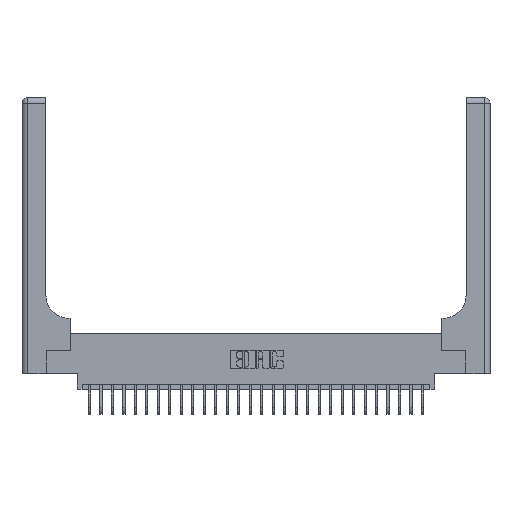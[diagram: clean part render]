
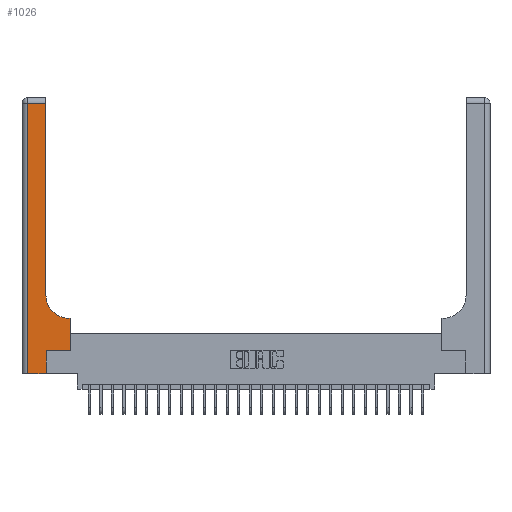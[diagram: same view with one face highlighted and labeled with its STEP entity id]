
A CAD part, top view. The second image highlights one B-rep face of the part: STEP entity #1026.
In plain terms, the highlighted planar face has unit normal (0, 0, 1).
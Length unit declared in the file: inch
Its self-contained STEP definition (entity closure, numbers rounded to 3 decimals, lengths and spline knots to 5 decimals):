
#331 = EDGE_CURVE ( 'NONE', #27107, #9258, #3644, .T. ) ;
#975 = CARTESIAN_POINT ( 'NONE',  ( 0.26, 0.85, 0.37 ) ) ;
#1026 = ADVANCED_FACE ( 'NONE', ( #7082 ), #26937, .F. ) ;
#1306 = CARTESIAN_POINT ( 'NONE',  ( 0.528, 0.25, 0.37 ) ) ;
#1690 = CARTESIAN_POINT ( 'NONE',  ( 0., 2.94, 0.37 ) ) ;
#1977 = DIRECTION ( 'NONE',  ( 0., 1., 0. ) ) ;
#2472 = CARTESIAN_POINT ( 'NONE',  ( 0.265, 0.25, 0.37 ) ) ;
#2735 = ORIENTED_EDGE ( 'NONE', *, *, #331, .T. ) ;
#2894 = ORIENTED_EDGE ( 'NONE', *, *, #18799, .T. ) ;
#2970 = DIRECTION ( 'NONE',  ( -1., 0., 0. ) ) ;
#3071 = EDGE_CURVE ( 'NONE', #18480, #27107, #7790, .T. ) ;
#3644 = CIRCLE ( 'NONE', #4906, 0.25 ) ;
#4906 = AXIS2_PLACEMENT_3D ( 'NONE', #14392, #12033, #23158 ) ;
#5175 = CARTESIAN_POINT ( 'NONE',  ( 0.265, 0., 0.37 ) ) ;
#5927 = VECTOR ( 'NONE', #7418, 39.37008 ) ;
#6182 = VERTEX_POINT ( 'NONE', #6375 ) ;
#6375 = CARTESIAN_POINT ( 'NONE',  ( 0.265, 0., 0.37 ) ) ;
#6427 = CARTESIAN_POINT ( 'NONE',  ( 0.06, 0., 0.37 ) ) ;
#7082 = FACE_OUTER_BOUND ( 'NONE', #8009, .T. ) ;
#7418 = DIRECTION ( 'NONE',  ( 0., 1., 0. ) ) ;
#7531 = DIRECTION ( 'NONE',  ( 0., 0., -1. ) ) ;
#7692 = ORIENTED_EDGE ( 'NONE', *, *, #22414, .T. ) ;
#7784 = LINE ( 'NONE', #23981, #21418 ) ;
#7790 = LINE ( 'NONE', #20280, #20394 ) ;
#7985 = LINE ( 'NONE', #5175, #5927 ) ;
#8009 = EDGE_LOOP ( 'NONE', ( #28107, #18977, #25809, #2894, #25044, #7692, #16005, #24424, #2735 ) ) ;
#8267 = VERTEX_POINT ( 'NONE', #21131 ) ;
#8695 = DIRECTION ( 'NONE',  ( 0., -1., 0. ) ) ;
#9064 = VERTEX_POINT ( 'NONE', #6427 ) ;
#9258 = VERTEX_POINT ( 'NONE', #975 ) ;
#9367 = LINE ( 'NONE', #1690, #11394 ) ;
#9979 = CARTESIAN_POINT ( 'NONE',  ( 0.06, 2.94, 0.37 ) ) ;
#10474 = VECTOR ( 'NONE', #1977, 39.37008 ) ;
#10831 = VERTEX_POINT ( 'NONE', #20837 ) ;
#10921 = DIRECTION ( 'NONE',  ( 1., 0., 0. ) ) ;
#11394 = VECTOR ( 'NONE', #14892, 39.37008 ) ;
#11463 = VERTEX_POINT ( 'NONE', #9979 ) ;
#12001 = EDGE_CURVE ( 'NONE', #9258, #8267, #27906, .T. ) ;
#12033 = DIRECTION ( 'NONE',  ( 0., 0., -1. ) ) ;
#12632 = LINE ( 'NONE', #21747, #21855 ) ;
#13184 = CARTESIAN_POINT ( 'NONE',  ( 0.26, 3., 0.37 ) ) ;
#14049 = EDGE_CURVE ( 'NONE', #6182, #10831, #7985, .T. ) ;
#14392 = CARTESIAN_POINT ( 'NONE',  ( 0.51, 0.85, 0.37 ) ) ;
#14892 = DIRECTION ( 'NONE',  ( -1., 0., 0. ) ) ;
#16005 = ORIENTED_EDGE ( 'NONE', *, *, #27167, .T. ) ;
#16258 = CARTESIAN_POINT ( 'NONE',  ( 0.51, 0.6, 0.37 ) ) ;
#16285 = AXIS2_PLACEMENT_3D ( 'NONE', #18296, #7531, #27121 ) ;
#16824 = DIRECTION ( 'NONE',  ( 0., 1., 0. ) ) ;
#17018 = CARTESIAN_POINT ( 'NONE',  ( 0.528, 0.25, 0.37 ) ) ;
#18296 = CARTESIAN_POINT ( 'NONE',  ( 0., 3., 0.37 ) ) ;
#18480 = VERTEX_POINT ( 'NONE', #23336 ) ;
#18799 = EDGE_CURVE ( 'NONE', #9064, #6182, #7784, .T. ) ;
#18977 = ORIENTED_EDGE ( 'NONE', *, *, #21145, .T. ) ;
#20280 = CARTESIAN_POINT ( 'NONE',  ( 0.26, 0.6, 0.37 ) ) ;
#20394 = VECTOR ( 'NONE', #2970, 39.37008 ) ;
#20837 = CARTESIAN_POINT ( 'NONE',  ( 0.265, 0.25, 0.37 ) ) ;
#21032 = VECTOR ( 'NONE', #16824, 39.37008 ) ;
#21131 = CARTESIAN_POINT ( 'NONE',  ( 0.26, 2.94, 0.37 ) ) ;
#21145 = EDGE_CURVE ( 'NONE', #8267, #11463, #9367, .T. ) ;
#21418 = VECTOR ( 'NONE', #10921, 39.37008 ) ;
#21747 = CARTESIAN_POINT ( 'NONE',  ( 0.06, 3., 0.37 ) ) ;
#21855 = VECTOR ( 'NONE', #8695, 39.37008 ) ;
#21884 = VECTOR ( 'NONE', #26884, 39.37008 ) ;
#22414 = EDGE_CURVE ( 'NONE', #10831, #27521, #23587, .T. ) ;
#23158 = DIRECTION ( 'NONE',  ( 1., 0., 0. ) ) ;
#23297 = EDGE_CURVE ( 'NONE', #11463, #9064, #12632, .T. ) ;
#23336 = CARTESIAN_POINT ( 'NONE',  ( 0.528, 0.6, 0.37 ) ) ;
#23587 = LINE ( 'NONE', #2472, #21884 ) ;
#23981 = CARTESIAN_POINT ( 'NONE',  ( 0., 0., 0.37 ) ) ;
#24424 = ORIENTED_EDGE ( 'NONE', *, *, #3071, .T. ) ;
#25044 = ORIENTED_EDGE ( 'NONE', *, *, #14049, .T. ) ;
#25809 = ORIENTED_EDGE ( 'NONE', *, *, #23297, .T. ) ;
#26474 = LINE ( 'NONE', #17018, #21032 ) ;
#26884 = DIRECTION ( 'NONE',  ( 1., 0., 0. ) ) ;
#26937 = PLANE ( 'NONE',  #16285 ) ;
#27107 = VERTEX_POINT ( 'NONE', #16258 ) ;
#27121 = DIRECTION ( 'NONE',  ( -1., 0., 0. ) ) ;
#27167 = EDGE_CURVE ( 'NONE', #27521, #18480, #26474, .T. ) ;
#27521 = VERTEX_POINT ( 'NONE', #1306 ) ;
#27906 = LINE ( 'NONE', #13184, #10474 ) ;
#28107 = ORIENTED_EDGE ( 'NONE', *, *, #12001, .T. ) ;
